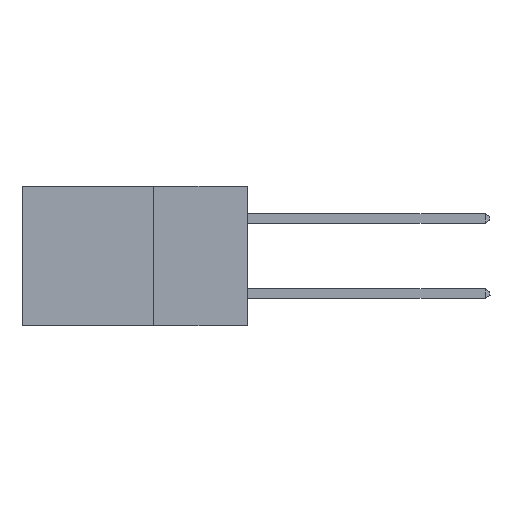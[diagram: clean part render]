
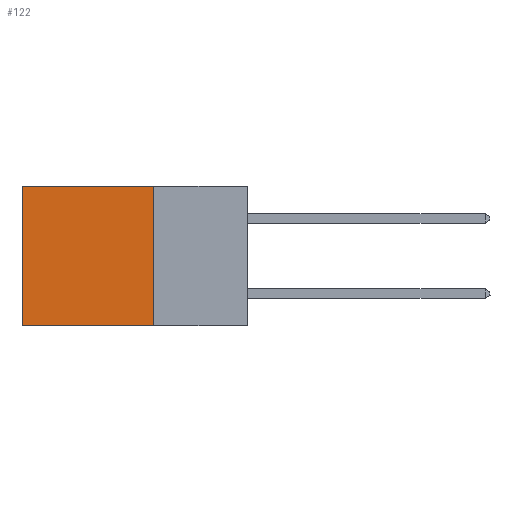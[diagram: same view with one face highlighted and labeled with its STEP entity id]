
A CAD part, left-side view. The second image highlights one B-rep face of the part: STEP entity #122.
In plain terms, the highlighted planar face has unit normal (-1, 0, 0).
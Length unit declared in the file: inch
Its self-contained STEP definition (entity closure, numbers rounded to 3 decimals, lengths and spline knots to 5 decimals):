
#122 = ADVANCED_FACE ( 'NONE', ( #14919 ), #15900, .F. ) ;
#521 = VERTEX_POINT ( 'NONE', #15616 ) ;
#921 = DIRECTION ( 'NONE',  ( 0., 0., -1. ) ) ;
#1229 = LINE ( 'NONE', #23698, #21702 ) ;
#2852 = CARTESIAN_POINT ( 'NONE',  ( 0.298, 0.25, 0. ) ) ;
#3675 = CARTESIAN_POINT ( 'NONE',  ( 0.298, 0.6, -0.37 ) ) ;
#5095 = ORIENTED_EDGE ( 'NONE', *, *, #19897, .F. ) ;
#5669 = EDGE_CURVE ( 'NONE', #521, #18805, #5715, .T. ) ;
#5715 = LINE ( 'NONE', #24675, #15788 ) ;
#5953 = CARTESIAN_POINT ( 'NONE',  ( 0.298, 0.25, 0. ) ) ;
#6144 = EDGE_LOOP ( 'NONE', ( #14581, #5095, #12679, #10827 ) ) ;
#6745 = CARTESIAN_POINT ( 'NONE',  ( 0.298, 0.25, 0. ) ) ;
#7777 = EDGE_CURVE ( 'NONE', #24250, #521, #1229, .T. ) ;
#10827 = ORIENTED_EDGE ( 'NONE', *, *, #7777, .T. ) ;
#11899 = DIRECTION ( 'NONE',  ( 0., 0., -1. ) ) ;
#12245 = DIRECTION ( 'NONE',  ( 1., 0., 0. ) ) ;
#12679 = ORIENTED_EDGE ( 'NONE', *, *, #24938, .F. ) ;
#14581 = ORIENTED_EDGE ( 'NONE', *, *, #5669, .T. ) ;
#14604 = CARTESIAN_POINT ( 'NONE',  ( 0.298, 0.25, -0.37 ) ) ;
#14919 = FACE_OUTER_BOUND ( 'NONE', #6144, .T. ) ;
#15209 = VECTOR ( 'NONE', #17325, 39.37008 ) ;
#15616 = CARTESIAN_POINT ( 'NONE',  ( 0.298, 0.6, 0. ) ) ;
#15788 = VECTOR ( 'NONE', #16931, 39.37008 ) ;
#15900 = PLANE ( 'NONE',  #22912 ) ;
#16931 = DIRECTION ( 'NONE',  ( 0., 0., -1. ) ) ;
#17102 = LINE ( 'NONE', #14604, #15209 ) ;
#17325 = DIRECTION ( 'NONE',  ( 0., 1., 0. ) ) ;
#18474 = VERTEX_POINT ( 'NONE', #20913 ) ;
#18805 = VERTEX_POINT ( 'NONE', #3675 ) ;
#19897 = EDGE_CURVE ( 'NONE', #18474, #18805, #17102, .T. ) ;
#20654 = VECTOR ( 'NONE', #921, 39.37008 ) ;
#20913 = CARTESIAN_POINT ( 'NONE',  ( 0.298, 0.25, -0.37 ) ) ;
#21702 = VECTOR ( 'NONE', #23873, 39.37008 ) ;
#22912 = AXIS2_PLACEMENT_3D ( 'NONE', #5953, #12245, #11899 ) ;
#23465 = LINE ( 'NONE', #2852, #20654 ) ;
#23698 = CARTESIAN_POINT ( 'NONE',  ( 0.298, 0.25, 0. ) ) ;
#23873 = DIRECTION ( 'NONE',  ( 0., 1., 0. ) ) ;
#24250 = VERTEX_POINT ( 'NONE', #6745 ) ;
#24675 = CARTESIAN_POINT ( 'NONE',  ( 0.298, 0.6, 0. ) ) ;
#24938 = EDGE_CURVE ( 'NONE', #24250, #18474, #23465, .T. ) ;
